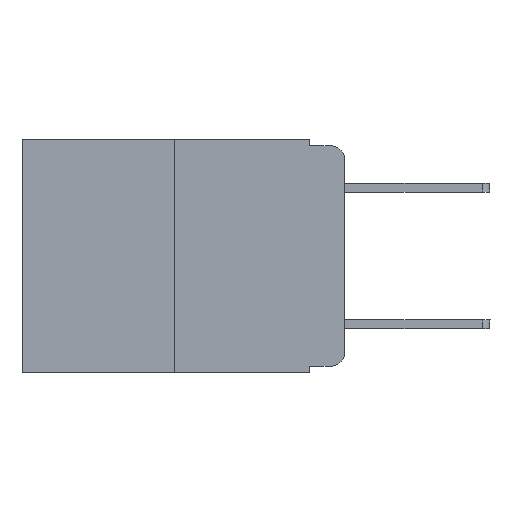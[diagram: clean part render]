
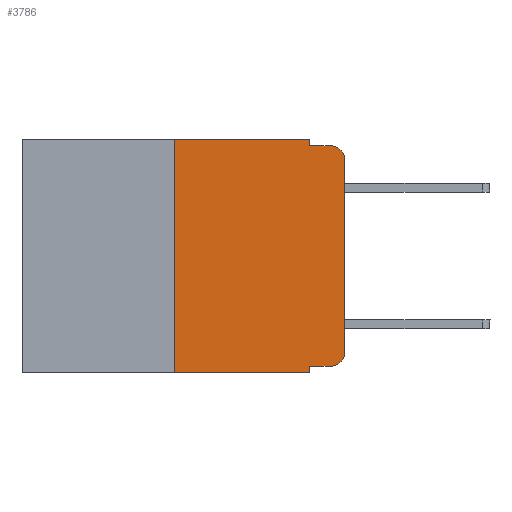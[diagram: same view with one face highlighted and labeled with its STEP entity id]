
A CAD part, left-side view. The second image highlights one B-rep face of the part: STEP entity #3786.
In plain terms, the highlighted planar face has unit normal (-1, 0, 0).
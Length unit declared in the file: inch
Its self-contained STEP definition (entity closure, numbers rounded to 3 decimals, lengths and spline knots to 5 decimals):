
#61 = EDGE_CURVE ( 'NONE', #8927, #975, #7729, .T. ) ;
#282 = CARTESIAN_POINT ( 'NONE',  ( 0., 0., -0.03 ) ) ;
#361 = PLANE ( 'NONE',  #2721 ) ;
#476 = CARTESIAN_POINT ( 'NONE',  ( 0., 0.02, -0.313 ) ) ;
#874 = DIRECTION ( 'NONE',  ( 0., 0., -1. ) ) ;
#975 = VERTEX_POINT ( 'NONE', #282 ) ;
#1127 = ORIENTED_EDGE ( 'NONE', *, *, #3211, .F. ) ;
#1207 = VERTEX_POINT ( 'NONE', #9442 ) ;
#1371 = LINE ( 'NONE', #4900, #6371 ) ;
#1525 = CARTESIAN_POINT ( 'NONE',  ( 0., 0.473, 0. ) ) ;
#1661 = DIRECTION ( 'NONE',  ( 0., 0., 1. ) ) ;
#1712 = CIRCLE ( 'NONE', #5348, 0.02 ) ;
#1773 = ORIENTED_EDGE ( 'NONE', *, *, #9252, .T. ) ;
#2038 = DIRECTION ( 'NONE',  ( -1., 0., 0. ) ) ;
#2091 = AXIS2_PLACEMENT_3D ( 'NONE', #6252, #2038, #9048 ) ;
#2125 = CARTESIAN_POINT ( 'NONE',  ( 0., 0.051, -0.333 ) ) ;
#2240 = VECTOR ( 'NONE', #874, 39.37008 ) ;
#2408 = DIRECTION ( 'NONE',  ( 0., 0., 1. ) ) ;
#2617 = LINE ( 'NONE', #6139, #8591 ) ;
#2646 = CARTESIAN_POINT ( 'NONE',  ( 0., 0.051, 0. ) ) ;
#2652 = ORIENTED_EDGE ( 'NONE', *, *, #5271, .F. ) ;
#2721 = AXIS2_PLACEMENT_3D ( 'NONE', #4708, #9894, #5507 ) ;
#2938 = FACE_OUTER_BOUND ( 'NONE', #5425, .T. ) ;
#3084 = CARTESIAN_POINT ( 'NONE',  ( 0., 0.25, -0.343 ) ) ;
#3103 = DIRECTION ( 'NONE',  ( 0., 0., -1. ) ) ;
#3211 = EDGE_CURVE ( 'NONE', #8017, #8763, #9993, .T. ) ;
#3273 = CARTESIAN_POINT ( 'NONE',  ( 0., 0.473, -0.343 ) ) ;
#3328 = DIRECTION ( 'NONE',  ( 0., -1., 0. ) ) ;
#3497 = VERTEX_POINT ( 'NONE', #3084 ) ;
#3786 = ADVANCED_FACE ( 'NONE', ( #2938 ), #361, .F. ) ;
#3802 = CARTESIAN_POINT ( 'NONE',  ( 0., 0.25, 0. ) ) ;
#4141 = DIRECTION ( 'NONE',  ( -1., 0., 0. ) ) ;
#4149 = CARTESIAN_POINT ( 'NONE',  ( 0., 0.02, -0.01 ) ) ;
#4210 = VERTEX_POINT ( 'NONE', #3802 ) ;
#4334 = CARTESIAN_POINT ( 'NONE',  ( 0., 0., 0. ) ) ;
#4377 = DIRECTION ( 'NONE',  ( 0., -1., 0. ) ) ;
#4427 = EDGE_CURVE ( 'NONE', #3497, #1207, #6772, .T. ) ;
#4506 = ORIENTED_EDGE ( 'NONE', *, *, #7064, .T. ) ;
#4708 = CARTESIAN_POINT ( 'NONE',  ( 0., 0.473, 0. ) ) ;
#4883 = EDGE_CURVE ( 'NONE', #10770, #8017, #8486, .T. ) ;
#4900 = CARTESIAN_POINT ( 'NONE',  ( 0., 0.25, 0. ) ) ;
#4992 = DIRECTION ( 'NONE',  ( 0., -1., 0. ) ) ;
#5170 = CARTESIAN_POINT ( 'NONE',  ( 0., 0.02, -0.333 ) ) ;
#5264 = ORIENTED_EDGE ( 'NONE', *, *, #5768, .F. ) ;
#5271 = EDGE_CURVE ( 'NONE', #3497, #4210, #1371, .T. ) ;
#5348 = AXIS2_PLACEMENT_3D ( 'NONE', #476, #4141, #3103 ) ;
#5425 = EDGE_LOOP ( 'NONE', ( #9290, #6868, #1127, #6590, #8586, #2652, #9895, #5264, #4506, #1773 ) ) ;
#5507 = DIRECTION ( 'NONE',  ( 0., 0., -1. ) ) ;
#5768 = EDGE_CURVE ( 'NONE', #8176, #1207, #6225, .T. ) ;
#5841 = LINE ( 'NONE', #1525, #11158 ) ;
#6118 = VECTOR ( 'NONE', #1661, 39.37008 ) ;
#6139 = CARTESIAN_POINT ( 'NONE',  ( 0., 0.051, -0.333 ) ) ;
#6225 = LINE ( 'NONE', #2646, #2240 ) ;
#6252 = CARTESIAN_POINT ( 'NONE',  ( 0., 0.02, -0.03 ) ) ;
#6363 = VECTOR ( 'NONE', #8260, 39.37008 ) ;
#6371 = VECTOR ( 'NONE', #2408, 39.37008 ) ;
#6590 = ORIENTED_EDGE ( 'NONE', *, *, #4883, .F. ) ;
#6772 = LINE ( 'NONE', #3273, #8172 ) ;
#6868 = ORIENTED_EDGE ( 'NONE', *, *, #8638, .T. ) ;
#7064 = EDGE_CURVE ( 'NONE', #8176, #10200, #2617, .T. ) ;
#7300 = CIRCLE ( 'NONE', #2091, 0.02 ) ;
#7407 = CARTESIAN_POINT ( 'NONE',  ( 0., 0.051, -0.01 ) ) ;
#7528 = EDGE_CURVE ( 'NONE', #4210, #10770, #5841, .T. ) ;
#7729 = LINE ( 'NONE', #4334, #6118 ) ;
#7916 = CARTESIAN_POINT ( 'NONE',  ( 0., 0.051, 0. ) ) ;
#8017 = VERTEX_POINT ( 'NONE', #10477 ) ;
#8172 = VECTOR ( 'NONE', #4992, 39.37008 ) ;
#8176 = VERTEX_POINT ( 'NONE', #2125 ) ;
#8260 = DIRECTION ( 'NONE',  ( 0., 0., -1. ) ) ;
#8486 = LINE ( 'NONE', #9298, #6363 ) ;
#8586 = ORIENTED_EDGE ( 'NONE', *, *, #7528, .F. ) ;
#8591 = VECTOR ( 'NONE', #4377, 39.37008 ) ;
#8638 = EDGE_CURVE ( 'NONE', #975, #8763, #7300, .T. ) ;
#8745 = CARTESIAN_POINT ( 'NONE',  ( 0., 0., -0.313 ) ) ;
#8763 = VERTEX_POINT ( 'NONE', #4149 ) ;
#8927 = VERTEX_POINT ( 'NONE', #8745 ) ;
#9048 = DIRECTION ( 'NONE',  ( 0., 0., -1. ) ) ;
#9252 = EDGE_CURVE ( 'NONE', #10200, #8927, #1712, .T. ) ;
#9290 = ORIENTED_EDGE ( 'NONE', *, *, #61, .T. ) ;
#9298 = CARTESIAN_POINT ( 'NONE',  ( 0., 0.051, 0. ) ) ;
#9442 = CARTESIAN_POINT ( 'NONE',  ( 0., 0.051, -0.343 ) ) ;
#9894 = DIRECTION ( 'NONE',  ( 1., 0., 0. ) ) ;
#9895 = ORIENTED_EDGE ( 'NONE', *, *, #4427, .T. ) ;
#9993 = LINE ( 'NONE', #7407, #10895 ) ;
#10200 = VERTEX_POINT ( 'NONE', #5170 ) ;
#10477 = CARTESIAN_POINT ( 'NONE',  ( 0., 0.051, -0.01 ) ) ;
#10770 = VERTEX_POINT ( 'NONE', #7916 ) ;
#10895 = VECTOR ( 'NONE', #10896, 39.37008 ) ;
#10896 = DIRECTION ( 'NONE',  ( 0., -1., 0. ) ) ;
#11158 = VECTOR ( 'NONE', #3328, 39.37008 ) ;
